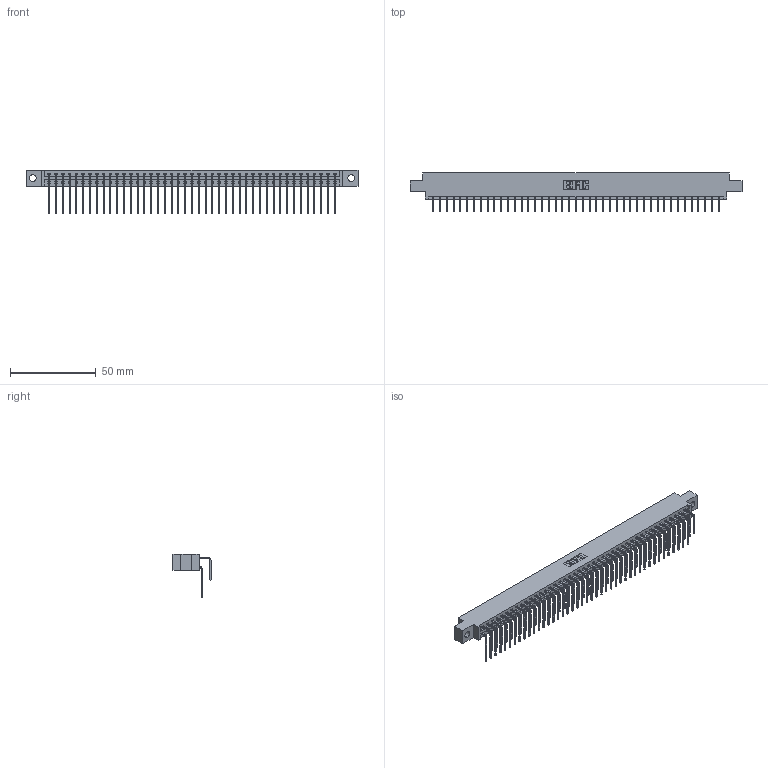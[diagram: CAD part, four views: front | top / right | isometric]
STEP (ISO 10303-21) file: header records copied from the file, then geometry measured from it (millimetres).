
FILE_DESCRIPTION (( 'STEP AP203' ), '1' );
FILE_NAME ('387-086-558-804.STEP', '2019-10-23T04:30:13', ( '' ), ( '' ), 'SwSTEP 2.0', 'SolidWorks 2016', '' );
FILE_SCHEMA (( 'CONFIG_CONTROL_DESIGN' ));
Length unit declared in the file: inch
Products named in the file (4): 337 Part_0.170 Offset - 0.156 Dia-TH; 387-086-558-804; 345-292-001_558 Tail - 2; 345-292-001_558 559 Tail - 1
Assembly tree (87 placements, depth 2):
  387-086-558-804
    337 Part_0.170 Offset - 0.156 Dia-TH
    345-292-001_558 559 Tail - 1  x43
    345-292-001_558 Tail - 2  x43
Bounding box: 193.4 x 22.17 x 25.53 mm (x, y, z)
Volume: 20685.6 mm3; surface area: 25791.2 mm2
Topology: 87 solids, 87 shells, 4934 faces, 14685 edges, 9674 vertices
Faces by surface type: plane 3514, cylinder 1420
Entity records: 35129 total; most frequent: CARTESIAN_POINT 5965, ORIENTED_EDGE 5850, DIRECTION 5053, EDGE_CURVE 2925, LINE 2757, VECTOR 2757, VERTEX_POINT 1946, AXIS2_PLACEMENT_3D 1148
